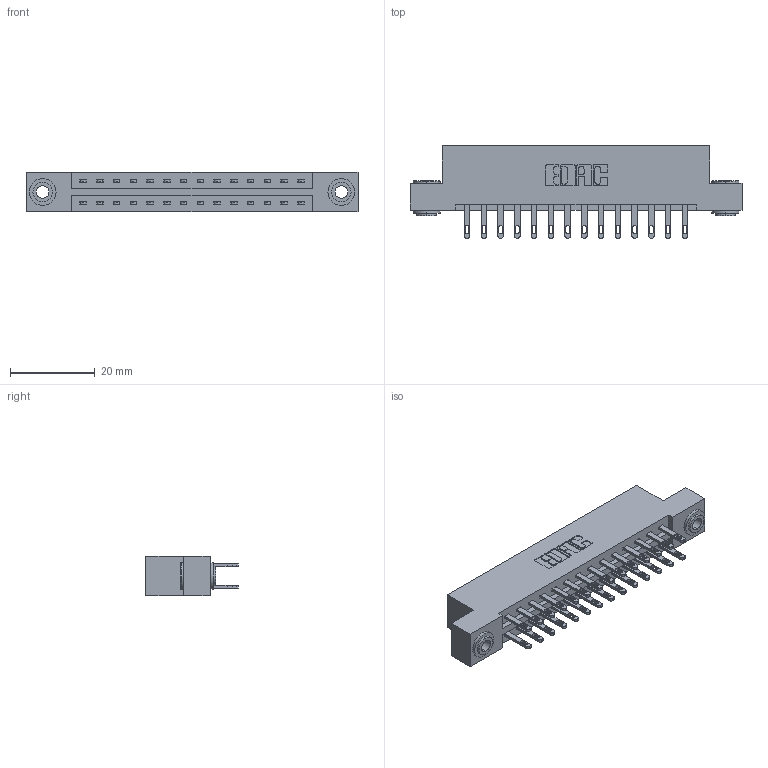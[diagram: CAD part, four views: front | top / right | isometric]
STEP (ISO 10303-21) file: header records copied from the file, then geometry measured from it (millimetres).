
FILE_DESCRIPTION (( 'STEP AP203' ), '1' );
FILE_NAME ('337-028-500-203.STEP', '2018-08-06T08:48:51', ( '' ), ( '' ), 'SwSTEP 2.0', 'SolidWorks 2016', '' );
FILE_SCHEMA (( 'CONFIG_CONTROL_DESIGN' ));
Length unit declared in the file: inch
Products named in the file (4): 337 Part_Flush Mounting Lugs - 0.156 Dia-TH; 345-292-001_345-293-100; 345-250-002_345-250-002-102; 337-028-500-203
Assembly tree (31 placements, depth 2):
  337-028-500-203
    337 Part_Flush Mounting Lugs - 0.156 Dia-TH
    345-292-001_345-293-100  x28
    345-250-002_345-250-002-102  x2
Bounding box: 78.49 x 21.85 x 9.4 mm (x, y, z)
Volume: 8003.7 mm3; surface area: 9311.3 mm2
Topology: 31 solids, 31 shells, 1552 faces, 4671 edges, 3110 vertices
Faces by surface type: plane 976, cylinder 568, cone 8
Entity records: 15056 total; most frequent: CARTESIAN_POINT 2533, ORIENTED_EDGE 2462, DIRECTION 2241, EDGE_CURVE 1231, VECTOR 1075, LINE 1075, VERTEX_POINT 818, AXIS2_PLACEMENT_3D 583
